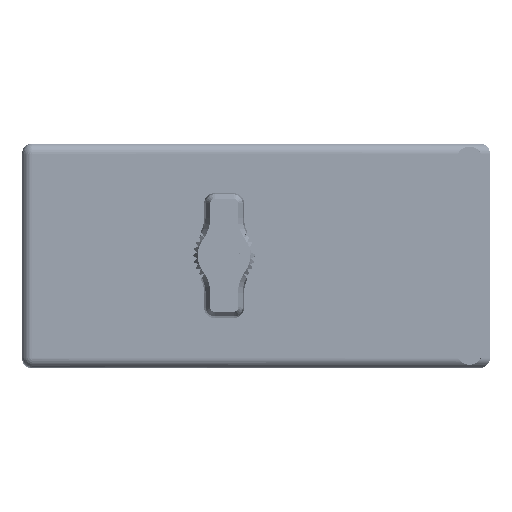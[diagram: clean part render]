
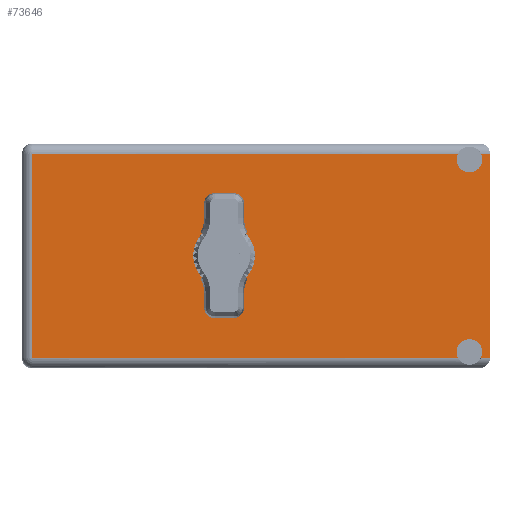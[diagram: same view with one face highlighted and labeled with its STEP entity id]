
A CAD part, top view. The second image highlights one B-rep face of the part: STEP entity #73646.
In plain terms, the highlighted face is planar.
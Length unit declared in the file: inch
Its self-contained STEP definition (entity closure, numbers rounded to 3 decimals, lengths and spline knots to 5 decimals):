
#969 = VERTEX_POINT ( 'NONE', #49838 ) ;
#1192 = EDGE_LOOP ( 'NONE', ( #62149, #82466, #19829, #69665, #18739, #27189, #89777, #90927, #16687, #13231 ) ) ;
#1200 = VERTEX_POINT ( 'NONE', #63200 ) ;
#2332 = VERTEX_POINT ( 'NONE', #16634 ) ;
#2568 = LINE ( 'NONE', #90107, #54093 ) ;
#3141 = EDGE_LOOP ( 'NONE', ( #59851, #35925 ) ) ;
#7162 = DIRECTION ( 'NONE',  ( 0., 0., 1. ) ) ;
#8525 = LINE ( 'NONE', #96093, #100958 ) ;
#9125 = AXIS2_PLACEMENT_3D ( 'NONE', #90295, #89550, #21338 ) ;
#9237 = CARTESIAN_POINT ( 'NONE',  ( 0.07, 2.03, -0.07 ) ) ;
#9320 = CARTESIAN_POINT ( 'NONE',  ( 3.05, 2.03, -0.109 ) ) ;
#10468 = AXIS2_PLACEMENT_3D ( 'NONE', #9320, #83134, #15624 ) ;
#11272 = EDGE_CURVE ( 'NONE', #87082, #36106, #8525, .T. ) ;
#13231 = ORIENTED_EDGE ( 'NONE', *, *, #79188, .T. ) ;
#15208 = DIRECTION ( 'NONE',  ( -1., 0., 0. ) ) ;
#15624 = DIRECTION ( 'NONE',  ( 0., 0., 1. ) ) ;
#16634 = CARTESIAN_POINT ( 'NONE',  ( 1.3775, 2.03, -0.935 ) ) ;
#16687 = ORIENTED_EDGE ( 'NONE', *, *, #97507, .T. ) ;
#17567 = CIRCLE ( 'NONE', #79361, 0.0875 ) ;
#17719 = VERTEX_POINT ( 'NONE', #80395 ) ;
#18739 = ORIENTED_EDGE ( 'NONE', *, *, #11272, .F. ) ;
#19339 = CARTESIAN_POINT ( 'NONE',  ( 2.97167, 2.03, -0.07 ) ) ;
#19507 = AXIS2_PLACEMENT_3D ( 'NONE', #46065, #105027, #54558 ) ;
#19829 = ORIENTED_EDGE ( 'NONE', *, *, #29591, .F. ) ;
#20228 = AXIS2_PLACEMENT_3D ( 'NONE', #93857, #76545, #101631 ) ;
#21338 = DIRECTION ( 'NONE',  ( 0., 0., 1. ) ) ;
#21414 = EDGE_CURVE ( 'NONE', #87082, #1200, #79308, .T. ) ;
#27189 = ORIENTED_EDGE ( 'NONE', *, *, #21414, .T. ) ;
#28025 = VERTEX_POINT ( 'NONE', #19339 ) ;
#29591 = EDGE_CURVE ( 'NONE', #17719, #95151, #17567, .T. ) ;
#33168 = CARTESIAN_POINT ( 'NONE',  ( 1.3775, 2.03, -0.765 ) ) ;
#33763 = VERTEX_POINT ( 'NONE', #104741 ) ;
#35925 = ORIENTED_EDGE ( 'NONE', *, *, #91849, .F. ) ;
#36106 = VERTEX_POINT ( 'NONE', #43814 ) ;
#36310 = CIRCLE ( 'NONE', #10468, 0.0875 ) ;
#36423 = DIRECTION ( 'NONE',  ( 0., 0., 1. ) ) ;
#37309 = FACE_OUTER_BOUND ( 'NONE', #1192, .T. ) ;
#40726 = VECTOR ( 'NONE', #7162, 39.37008 ) ;
#40786 = CARTESIAN_POINT ( 'NONE',  ( 0.07, 2.03, -1.53 ) ) ;
#41160 = LINE ( 'NONE', #51588, #51748 ) ;
#41296 = DIRECTION ( 'NONE',  ( 0., 1., 0. ) ) ;
#42113 = CARTESIAN_POINT ( 'NONE',  ( 0., 2.03, -1.46 ) ) ;
#43500 = CARTESIAN_POINT ( 'NONE',  ( 2.97167, 2.03, -1.46 ) ) ;
#43814 = CARTESIAN_POINT ( 'NONE',  ( 3.19, 2.03, -0.07 ) ) ;
#44518 = VERTEX_POINT ( 'NONE', #9237 ) ;
#44798 = DIRECTION ( 'NONE',  ( 1., 0., 0. ) ) ;
#46065 = CARTESIAN_POINT ( 'NONE',  ( 0., 2.03, -1.53 ) ) ;
#47516 = PLANE ( 'NONE',  #19507 ) ;
#49593 = CIRCLE ( 'NONE', #86744, 0.17 ) ;
#49838 = CARTESIAN_POINT ( 'NONE',  ( 0.07, 2.03, -1.46 ) ) ;
#51133 = VERTEX_POINT ( 'NONE', #43500 ) ;
#51541 = CIRCLE ( 'NONE', #20228, 0.0875 ) ;
#51588 = CARTESIAN_POINT ( 'NONE',  ( 3.19, 2.03, -0.07 ) ) ;
#51748 = VECTOR ( 'NONE', #76611, 39.37008 ) ;
#51788 = DIRECTION ( 'NONE',  ( 0., 1., 0. ) ) ;
#54093 = VECTOR ( 'NONE', #15208, 39.37008 ) ;
#54558 = DIRECTION ( 'NONE',  ( 0., 0., 1. ) ) ;
#54950 = EDGE_CURVE ( 'NONE', #17719, #36106, #108932, .T. ) ;
#56570 = CARTESIAN_POINT ( 'NONE',  ( 3.05, 2.03, -0.1965 ) ) ;
#59851 = ORIENTED_EDGE ( 'NONE', *, *, #89406, .F. ) ;
#59987 = CARTESIAN_POINT ( 'NONE',  ( 3.05, 2.03, -0.109 ) ) ;
#61759 = EDGE_CURVE ( 'NONE', #44518, #28025, #41160, .T. ) ;
#62149 = ORIENTED_EDGE ( 'NONE', *, *, #61759, .T. ) ;
#63200 = CARTESIAN_POINT ( 'NONE',  ( 3.12833, 2.03, -1.46 ) ) ;
#64359 = CARTESIAN_POINT ( 'NONE',  ( 1.3775, 2.03, -0.595 ) ) ;
#66350 = DIRECTION ( 'NONE',  ( 0., 0., 1. ) ) ;
#67634 = FACE_BOUND ( 'NONE', #3141, .T. ) ;
#69184 = DIRECTION ( 'NONE',  ( 0., 1., 0. ) ) ;
#69370 = CARTESIAN_POINT ( 'NONE',  ( 3.19, 2.03, -1.46 ) ) ;
#69665 = ORIENTED_EDGE ( 'NONE', *, *, #54950, .T. ) ;
#70087 = VECTOR ( 'NONE', #100368, 39.37008 ) ;
#73043 = CIRCLE ( 'NONE', #101756, 0.0875 ) ;
#73646 = ADVANCED_FACE ( 'NONE', ( #67634, #37309 ), #47516, .T. ) ;
#76545 = DIRECTION ( 'NONE',  ( 0., 1., 0. ) ) ;
#76611 = DIRECTION ( 'NONE',  ( 1., 0., 0. ) ) ;
#77162 = CARTESIAN_POINT ( 'NONE',  ( 3.05, 2.03, -1.421 ) ) ;
#79188 = EDGE_CURVE ( 'NONE', #969, #44518, #93474, .T. ) ;
#79308 = LINE ( 'NONE', #42113, #70087 ) ;
#79361 = AXIS2_PLACEMENT_3D ( 'NONE', #59987, #69184, #36423 ) ;
#80395 = CARTESIAN_POINT ( 'NONE',  ( 3.12833, 2.03, -0.07 ) ) ;
#82466 = ORIENTED_EDGE ( 'NONE', *, *, #99808, .F. ) ;
#83134 = DIRECTION ( 'NONE',  ( 0., 1., 0. ) ) ;
#85642 = DIRECTION ( 'NONE',  ( 0., 0., 1. ) ) ;
#86489 = VECTOR ( 'NONE', #44798, 39.37008 ) ;
#86744 = AXIS2_PLACEMENT_3D ( 'NONE', #33168, #41296, #66350 ) ;
#86787 = CARTESIAN_POINT ( 'NONE',  ( 3.19, 2.03, -0.07 ) ) ;
#87082 = VERTEX_POINT ( 'NONE', #69370 ) ;
#89406 = EDGE_CURVE ( 'NONE', #104950, #2332, #49593, .T. ) ;
#89550 = DIRECTION ( 'NONE',  ( 0., 1., 0. ) ) ;
#89777 = ORIENTED_EDGE ( 'NONE', *, *, #91059, .F. ) ;
#90107 = CARTESIAN_POINT ( 'NONE',  ( 0., 2.03, -1.46 ) ) ;
#90295 = CARTESIAN_POINT ( 'NONE',  ( 1.3775, 2.03, -0.765 ) ) ;
#90927 = ORIENTED_EDGE ( 'NONE', *, *, #97075, .F. ) ;
#91059 = EDGE_CURVE ( 'NONE', #33763, #1200, #73043, .T. ) ;
#91849 = EDGE_CURVE ( 'NONE', #2332, #104950, #108485, .T. ) ;
#93474 = LINE ( 'NONE', #40786, #40726 ) ;
#93857 = CARTESIAN_POINT ( 'NONE',  ( 3.05, 2.03, -1.421 ) ) ;
#94591 = DIRECTION ( 'NONE',  ( 0., 0., 1. ) ) ;
#95151 = VERTEX_POINT ( 'NONE', #56570 ) ;
#96093 = CARTESIAN_POINT ( 'NONE',  ( 3.19, 2.03, 0. ) ) ;
#97075 = EDGE_CURVE ( 'NONE', #51133, #33763, #51541, .T. ) ;
#97507 = EDGE_CURVE ( 'NONE', #51133, #969, #2568, .T. ) ;
#99808 = EDGE_CURVE ( 'NONE', #95151, #28025, #36310, .T. ) ;
#100368 = DIRECTION ( 'NONE',  ( -1., 0., 0. ) ) ;
#100958 = VECTOR ( 'NONE', #94591, 39.37008 ) ;
#101631 = DIRECTION ( 'NONE',  ( 0., 0., 1. ) ) ;
#101756 = AXIS2_PLACEMENT_3D ( 'NONE', #77162, #51788, #85642 ) ;
#104741 = CARTESIAN_POINT ( 'NONE',  ( 3.05, 2.03, -1.3335 ) ) ;
#104950 = VERTEX_POINT ( 'NONE', #64359 ) ;
#105027 = DIRECTION ( 'NONE',  ( 0., 1., 0. ) ) ;
#108485 = CIRCLE ( 'NONE', #9125, 0.17 ) ;
#108932 = LINE ( 'NONE', #86787, #86489 ) ;
